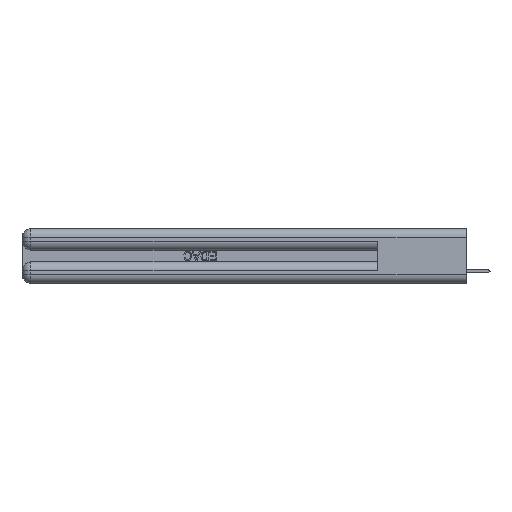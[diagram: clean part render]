
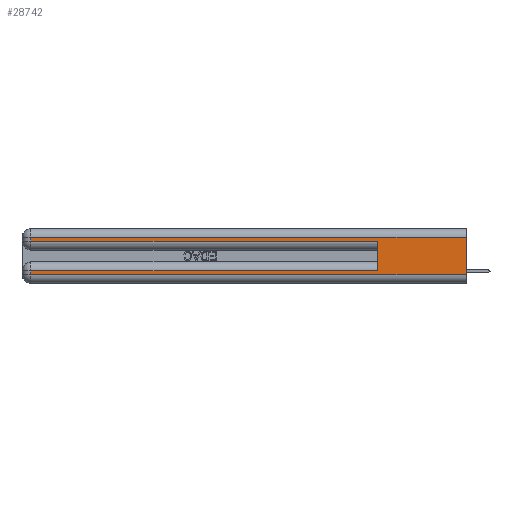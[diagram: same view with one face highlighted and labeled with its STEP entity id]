
A CAD part, left-side view. The second image highlights one B-rep face of the part: STEP entity #28742.
In plain terms, the highlighted planar face has unit normal (-1, 0, 0).
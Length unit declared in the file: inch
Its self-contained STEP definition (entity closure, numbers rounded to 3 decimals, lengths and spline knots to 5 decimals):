
#1099 = VERTEX_POINT ( 'NONE', #42945 ) ;
#2835 = CARTESIAN_POINT ( 'NONE',  ( 0., 2.94, 0.085 ) ) ;
#3092 = VERTEX_POINT ( 'NONE', #2835 ) ;
#3813 = FACE_OUTER_BOUND ( 'NONE', #7660, .T. ) ;
#3881 = DIRECTION ( 'NONE',  ( 1., 0., 0. ) ) ;
#3979 = EDGE_CURVE ( 'NONE', #21688, #13850, #40524, .T. ) ;
#4476 = CARTESIAN_POINT ( 'NONE',  ( 0., 0.6, 0.085 ) ) ;
#4585 = LINE ( 'NONE', #16981, #34889 ) ;
#5479 = VECTOR ( 'NONE', #7394, 39.37008 ) ;
#6278 = CARTESIAN_POINT ( 'NONE',  ( 0., 0., 0.085 ) ) ;
#7394 = DIRECTION ( 'NONE',  ( 0., 0., 1. ) ) ;
#7435 = CARTESIAN_POINT ( 'NONE',  ( 0., 0., 0.285 ) ) ;
#7660 = EDGE_LOOP ( 'NONE', ( #30358, #36469, #44551, #11773, #46887, #22079, #17290, #45834 ) ) ;
#8065 = LINE ( 'NONE', #7435, #40849 ) ;
#11181 = CARTESIAN_POINT ( 'NONE',  ( 0., 2.94, 0.06 ) ) ;
#11773 = ORIENTED_EDGE ( 'NONE', *, *, #44867, .T. ) ;
#13169 = LINE ( 'NONE', #22757, #38530 ) ;
#13338 = CARTESIAN_POINT ( 'NONE',  ( 0., 0., 0.37 ) ) ;
#13850 = VERTEX_POINT ( 'NONE', #42979 ) ;
#14069 = DIRECTION ( 'NONE',  ( 0., 1., 0. ) ) ;
#15355 = VECTOR ( 'NONE', #42640, 39.37008 ) ;
#16227 = DIRECTION ( 'NONE',  ( 0., 1., 0. ) ) ;
#16981 = CARTESIAN_POINT ( 'NONE',  ( 0., 0., 0.31 ) ) ;
#17290 = ORIENTED_EDGE ( 'NONE', *, *, #49884, .T. ) ;
#17829 = EDGE_CURVE ( 'NONE', #41012, #3092, #19150, .T. ) ;
#18132 = DIRECTION ( 'NONE',  ( 0., 0., -1. ) ) ;
#18220 = DIRECTION ( 'NONE',  ( 0., -1., 0. ) ) ;
#19150 = LINE ( 'NONE', #6278, #45717 ) ;
#19370 = CARTESIAN_POINT ( 'NONE',  ( 0., 0., 0.37 ) ) ;
#21688 = VERTEX_POINT ( 'NONE', #11181 ) ;
#22079 = ORIENTED_EDGE ( 'NONE', *, *, #17829, .T. ) ;
#22084 = AXIS2_PLACEMENT_3D ( 'NONE', #19370, #3881, #23351 ) ;
#22101 = EDGE_CURVE ( 'NONE', #40437, #1099, #4585, .T. ) ;
#22676 = EDGE_CURVE ( 'NONE', #1099, #49944, #13169, .T. ) ;
#22757 = CARTESIAN_POINT ( 'NONE',  ( 0., 2.94, 0.37 ) ) ;
#23351 = DIRECTION ( 'NONE',  ( 0., 0., -1. ) ) ;
#23841 = VERTEX_POINT ( 'NONE', #28191 ) ;
#24290 = CARTESIAN_POINT ( 'NONE',  ( 0., 2.94, 0.285 ) ) ;
#25025 = CARTESIAN_POINT ( 'NONE',  ( 0., 0., 0.31 ) ) ;
#26532 = DIRECTION ( 'NONE',  ( 0., 0., -1. ) ) ;
#28191 = CARTESIAN_POINT ( 'NONE',  ( 0., 0.6, 0.285 ) ) ;
#28742 = ADVANCED_FACE ( 'NONE', ( #3813 ), #31294, .F. ) ;
#28833 = EDGE_CURVE ( 'NONE', #40437, #13850, #29697, .T. ) ;
#29697 = LINE ( 'NONE', #13338, #41458 ) ;
#30358 = ORIENTED_EDGE ( 'NONE', *, *, #28833, .F. ) ;
#31294 = PLANE ( 'NONE',  #22084 ) ;
#34889 = VECTOR ( 'NONE', #14069, 39.37008 ) ;
#36469 = ORIENTED_EDGE ( 'NONE', *, *, #22101, .T. ) ;
#38530 = VECTOR ( 'NONE', #26532, 39.37008 ) ;
#40437 = VERTEX_POINT ( 'NONE', #25025 ) ;
#40524 = LINE ( 'NONE', #41899, #42963 ) ;
#40712 = LINE ( 'NONE', #50883, #15355 ) ;
#40849 = VECTOR ( 'NONE', #42679, 39.37008 ) ;
#41012 = VERTEX_POINT ( 'NONE', #4476 ) ;
#41316 = LINE ( 'NONE', #50714, #5479 ) ;
#41458 = VECTOR ( 'NONE', #18132, 39.37008 ) ;
#41899 = CARTESIAN_POINT ( 'NONE',  ( 0., 0., 0.06 ) ) ;
#42640 = DIRECTION ( 'NONE',  ( 0., 0., -1. ) ) ;
#42679 = DIRECTION ( 'NONE',  ( 0., -1., 0. ) ) ;
#42945 = CARTESIAN_POINT ( 'NONE',  ( 0., 2.94, 0.31 ) ) ;
#42963 = VECTOR ( 'NONE', #18220, 39.37008 ) ;
#42979 = CARTESIAN_POINT ( 'NONE',  ( 0., 0., 0.06 ) ) ;
#44551 = ORIENTED_EDGE ( 'NONE', *, *, #22676, .T. ) ;
#44867 = EDGE_CURVE ( 'NONE', #49944, #23841, #8065, .T. ) ;
#45717 = VECTOR ( 'NONE', #16227, 39.37008 ) ;
#45834 = ORIENTED_EDGE ( 'NONE', *, *, #3979, .T. ) ;
#46887 = ORIENTED_EDGE ( 'NONE', *, *, #49859, .F. ) ;
#49859 = EDGE_CURVE ( 'NONE', #41012, #23841, #41316, .T. ) ;
#49884 = EDGE_CURVE ( 'NONE', #3092, #21688, #40712, .T. ) ;
#49944 = VERTEX_POINT ( 'NONE', #24290 ) ;
#50714 = CARTESIAN_POINT ( 'NONE',  ( 0., 0.6, 0.145 ) ) ;
#50883 = CARTESIAN_POINT ( 'NONE',  ( 0., 2.94, 0.37 ) ) ;
